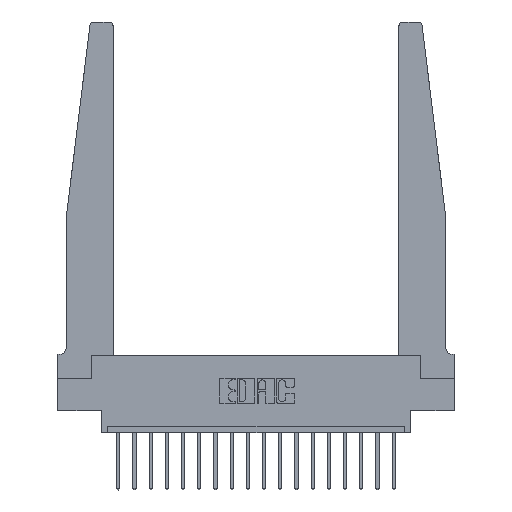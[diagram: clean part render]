
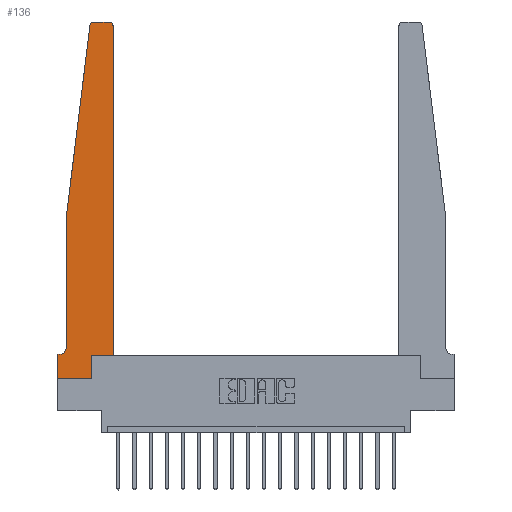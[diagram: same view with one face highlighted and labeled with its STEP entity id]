
A CAD part, top view. The second image highlights one B-rep face of the part: STEP entity #136.
In plain terms, the highlighted planar face has unit normal (0, 0, 1).
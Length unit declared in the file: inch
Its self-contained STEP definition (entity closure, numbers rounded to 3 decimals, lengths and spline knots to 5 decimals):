
#136 = ADVANCED_FACE ( 'NONE', ( #360 ), #9804, .T. ) ;
#180 = LINE ( 'NONE', #2735, #10837 ) ;
#277 = DIRECTION ( 'NONE',  ( 0., -1., 0. ) ) ;
#350 = VECTOR ( 'NONE', #4831, 39.37008 ) ;
#360 = FACE_OUTER_BOUND ( 'NONE', #5846, .T. ) ;
#370 = LINE ( 'NONE', #10345, #7046 ) ;
#757 = VERTEX_POINT ( 'NONE', #17399 ) ;
#1538 = DIRECTION ( 'NONE',  ( 1., 0., 0. ) ) ;
#1614 = ORIENTED_EDGE ( 'NONE', *, *, #8494, .T. ) ;
#2063 = VERTEX_POINT ( 'NONE', #11081 ) ;
#2174 = DIRECTION ( 'NONE',  ( 1., 0., 0. ) ) ;
#2720 = ORIENTED_EDGE ( 'NONE', *, *, #3989, .T. ) ;
#2735 = CARTESIAN_POINT ( 'NONE',  ( 0., 0., 0.37 ) ) ;
#2785 = EDGE_CURVE ( 'NONE', #18716, #8365, #14319, .T. ) ;
#3060 = CIRCLE ( 'NONE', #4720, 0.03 ) ;
#3418 = CARTESIAN_POINT ( 'NONE',  ( 0.425, 0.18, 0.37 ) ) ;
#3478 = DIRECTION ( 'NONE',  ( 0., 0., 1. ) ) ;
#3481 = VECTOR ( 'NONE', #2174, 39.37008 ) ;
#3594 = CARTESIAN_POINT ( 'NONE',  ( 0., 0., 0.37 ) ) ;
#3885 = CARTESIAN_POINT ( 'NONE',  ( 0.2605, 0.18, 0.37 ) ) ;
#3989 = EDGE_CURVE ( 'NONE', #12723, #18716, #17218, .T. ) ;
#4241 = EDGE_CURVE ( 'NONE', #6975, #7540, #12549, .T. ) ;
#4611 = DIRECTION ( 'NONE',  ( 0., 0., 1. ) ) ;
#4720 = AXIS2_PLACEMENT_3D ( 'NONE', #16229, #4611, #1538 ) ;
#4793 = AXIS2_PLACEMENT_3D ( 'NONE', #16844, #3478, #18435 ) ;
#4831 = DIRECTION ( 'NONE',  ( -1., 0., 0. ) ) ;
#5555 = CARTESIAN_POINT ( 'NONE',  ( 0.2605, 0., 0.37 ) ) ;
#5678 = CARTESIAN_POINT ( 'NONE',  ( 0.065, 0.2375, 0.37 ) ) ;
#5846 = EDGE_LOOP ( 'NONE', ( #19201, #11697, #2720, #11829, #12979, #17506, #8356, #9846, #19141, #13551, #1614, #11336 ) ) ;
#6070 = CARTESIAN_POINT ( 'NONE',  ( 0.065, 1.25, 0.37 ) ) ;
#6110 = EDGE_CURVE ( 'NONE', #12265, #6975, #180, .T. ) ;
#6265 = EDGE_CURVE ( 'NONE', #8365, #6837, #6974, .T. ) ;
#6540 = DIRECTION ( 'NONE',  ( 1., 0., 0. ) ) ;
#6726 = DIRECTION ( 'NONE',  ( 0., 0., 1. ) ) ;
#6837 = VERTEX_POINT ( 'NONE', #15295 ) ;
#6842 = LINE ( 'NONE', #3885, #13193 ) ;
#6974 = CIRCLE ( 'NONE', #16790, 0.05 ) ;
#6975 = VERTEX_POINT ( 'NONE', #12489 ) ;
#7041 = VECTOR ( 'NONE', #6540, 39.37008 ) ;
#7046 = VECTOR ( 'NONE', #10891, 39.37008 ) ;
#7051 = CARTESIAN_POINT ( 'NONE',  ( 0.065, 0.1875, 0.37 ) ) ;
#7072 = VERTEX_POINT ( 'NONE', #14446 ) ;
#7245 = CIRCLE ( 'NONE', #4793, 0.03 ) ;
#7540 = VERTEX_POINT ( 'NONE', #5555 ) ;
#7614 = CARTESIAN_POINT ( 'NONE',  ( 0.065, 1.25, 0.37 ) ) ;
#7772 = EDGE_CURVE ( 'NONE', #7072, #2063, #7245, .T. ) ;
#8356 = ORIENTED_EDGE ( 'NONE', *, *, #6110, .T. ) ;
#8365 = VERTEX_POINT ( 'NONE', #5678 ) ;
#8494 = EDGE_CURVE ( 'NONE', #757, #7072, #370, .T. ) ;
#8754 = DIRECTION ( 'NONE',  ( 0., -1., 0. ) ) ;
#9804 = PLANE ( 'NONE',  #18868 ) ;
#9846 = ORIENTED_EDGE ( 'NONE', *, *, #4241, .T. ) ;
#9931 = LINE ( 'NONE', #7051, #15107 ) ;
#9998 = DIRECTION ( 'NONE',  ( 0., 1., 0. ) ) ;
#10345 = CARTESIAN_POINT ( 'NONE',  ( 0.425, 0.18, 0.37 ) ) ;
#10837 = VECTOR ( 'NONE', #8754, 39.37008 ) ;
#10891 = DIRECTION ( 'NONE',  ( 0., 1., 0. ) ) ;
#10930 = CARTESIAN_POINT ( 'NONE',  ( 0.015, 0.2375, 0.37 ) ) ;
#11066 = CARTESIAN_POINT ( 'NONE',  ( 0., 0.1875, 0.37 ) ) ;
#11078 = EDGE_CURVE ( 'NONE', #15335, #12723, #3060, .T. ) ;
#11081 = CARTESIAN_POINT ( 'NONE',  ( 0.395, 2.75, 0.37 ) ) ;
#11336 = ORIENTED_EDGE ( 'NONE', *, *, #7772, .T. ) ;
#11697 = ORIENTED_EDGE ( 'NONE', *, *, #11078, .T. ) ;
#11829 = ORIENTED_EDGE ( 'NONE', *, *, #2785, .T. ) ;
#12225 = VERTEX_POINT ( 'NONE', #18696 ) ;
#12265 = VERTEX_POINT ( 'NONE', #14211 ) ;
#12322 = EDGE_CURVE ( 'NONE', #6837, #12265, #9931, .T. ) ;
#12415 = VECTOR ( 'NONE', #17954, 39.37008 ) ;
#12448 = VECTOR ( 'NONE', #277, 39.37008 ) ;
#12489 = CARTESIAN_POINT ( 'NONE',  ( 0., 0., 0.37 ) ) ;
#12549 = LINE ( 'NONE', #3594, #3481 ) ;
#12723 = VERTEX_POINT ( 'NONE', #16556 ) ;
#12979 = ORIENTED_EDGE ( 'NONE', *, *, #6265, .T. ) ;
#13193 = VECTOR ( 'NONE', #9998, 39.37008 ) ;
#13551 = ORIENTED_EDGE ( 'NONE', *, *, #18345, .T. ) ;
#13743 = DIRECTION ( 'NONE',  ( -1., 0., 0. ) ) ;
#13930 = DIRECTION ( 'NONE',  ( 0., 0., -1. ) ) ;
#14080 = EDGE_CURVE ( 'NONE', #7540, #12225, #6842, .T. ) ;
#14211 = CARTESIAN_POINT ( 'NONE',  ( 0., 0.1875, 0.37 ) ) ;
#14319 = LINE ( 'NONE', #7614, #12448 ) ;
#14446 = CARTESIAN_POINT ( 'NONE',  ( 0.425, 2.72, 0.37 ) ) ;
#15107 = VECTOR ( 'NONE', #17505, 39.37008 ) ;
#15234 = LINE ( 'NONE', #16928, #350 ) ;
#15295 = CARTESIAN_POINT ( 'NONE',  ( 0.015, 0.1875, 0.37 ) ) ;
#15335 = VERTEX_POINT ( 'NONE', #16795 ) ;
#16229 = CARTESIAN_POINT ( 'NONE',  ( 0.27653, 2.72, 0.37 ) ) ;
#16556 = CARTESIAN_POINT ( 'NONE',  ( 0.24675, 2.72367, 0.37 ) ) ;
#16790 = AXIS2_PLACEMENT_3D ( 'NONE', #10930, #13930, #13743 ) ;
#16795 = CARTESIAN_POINT ( 'NONE',  ( 0.27653, 2.75, 0.37 ) ) ;
#16844 = CARTESIAN_POINT ( 'NONE',  ( 0.395, 2.72, 0.37 ) ) ;
#16921 = LINE ( 'NONE', #3418, #7041 ) ;
#16928 = CARTESIAN_POINT ( 'NONE',  ( 0.25, 2.75, 0.37 ) ) ;
#17168 = DIRECTION ( 'NONE',  ( 1., 0., 0. ) ) ;
#17218 = LINE ( 'NONE', #19329, #12415 ) ;
#17399 = CARTESIAN_POINT ( 'NONE',  ( 0.425, 0.18, 0.37 ) ) ;
#17505 = DIRECTION ( 'NONE',  ( -1., 0., 0. ) ) ;
#17506 = ORIENTED_EDGE ( 'NONE', *, *, #12322, .T. ) ;
#17954 = DIRECTION ( 'NONE',  ( -0.122, -0.992, 0. ) ) ;
#18345 = EDGE_CURVE ( 'NONE', #12225, #757, #16921, .T. ) ;
#18435 = DIRECTION ( 'NONE',  ( 1., 0., 0. ) ) ;
#18696 = CARTESIAN_POINT ( 'NONE',  ( 0.2605, 0.18, 0.37 ) ) ;
#18716 = VERTEX_POINT ( 'NONE', #6070 ) ;
#18860 = EDGE_CURVE ( 'NONE', #2063, #15335, #15234, .T. ) ;
#18868 = AXIS2_PLACEMENT_3D ( 'NONE', #11066, #6726, #17168 ) ;
#19141 = ORIENTED_EDGE ( 'NONE', *, *, #14080, .T. ) ;
#19201 = ORIENTED_EDGE ( 'NONE', *, *, #18860, .T. ) ;
#19329 = CARTESIAN_POINT ( 'NONE',  ( 0.065, 1.25, 0.37 ) ) ;
